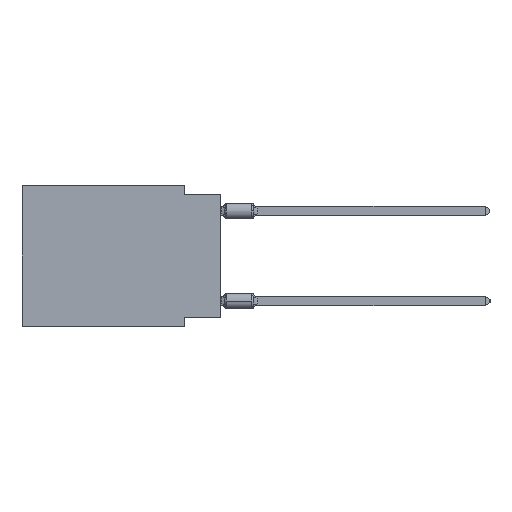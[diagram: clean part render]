
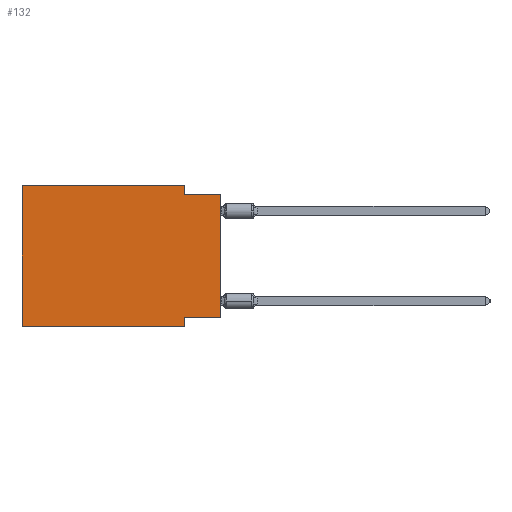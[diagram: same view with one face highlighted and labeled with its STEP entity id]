
A CAD part, left-side view. The second image highlights one B-rep face of the part: STEP entity #132.
In plain terms, the highlighted planar face has unit normal (-1, 0, 0).
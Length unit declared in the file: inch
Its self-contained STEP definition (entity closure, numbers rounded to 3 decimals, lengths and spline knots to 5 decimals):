
#132 = ADVANCED_FACE ( 'NONE', ( #26455 ), #16922, .F. ) ;
#209 = EDGE_CURVE ( 'NONE', #11832, #722, #6867, .T. ) ;
#321 = LINE ( 'NONE', #10527, #19018 ) ;
#358 = DIRECTION ( 'NONE',  ( 0., 0., -1. ) ) ;
#425 = CARTESIAN_POINT ( 'NONE',  ( 0., 0., -0.025 ) ) ;
#722 = VERTEX_POINT ( 'NONE', #29052 ) ;
#1105 = VECTOR ( 'NONE', #358, 39.37008 ) ;
#1753 = DIRECTION ( 'NONE',  ( 1., 0., 0. ) ) ;
#3013 = LINE ( 'NONE', #30524, #1105 ) ;
#3187 = CARTESIAN_POINT ( 'NONE',  ( 0., 0., -0.365 ) ) ;
#3414 = VERTEX_POINT ( 'NONE', #19768 ) ;
#3905 = CARTESIAN_POINT ( 'NONE',  ( 0., 0.55, 0. ) ) ;
#4203 = AXIS2_PLACEMENT_3D ( 'NONE', #3905, #1753, #29095 ) ;
#6547 = CARTESIAN_POINT ( 'NONE',  ( 0., 0.1, 0. ) ) ;
#6650 = ORIENTED_EDGE ( 'NONE', *, *, #29972, .F. ) ;
#6814 = ORIENTED_EDGE ( 'NONE', *, *, #30491, .F. ) ;
#6867 = LINE ( 'NONE', #6547, #7370 ) ;
#7124 = LINE ( 'NONE', #12048, #7965 ) ;
#7370 = VECTOR ( 'NONE', #11789, 39.37008 ) ;
#7598 = DIRECTION ( 'NONE',  ( 0., 0., 1. ) ) ;
#7965 = VECTOR ( 'NONE', #32156, 39.37008 ) ;
#8181 = ORIENTED_EDGE ( 'NONE', *, *, #19291, .F. ) ;
#8898 = VERTEX_POINT ( 'NONE', #12529 ) ;
#9011 = LINE ( 'NONE', #29116, #17925 ) ;
#10527 = CARTESIAN_POINT ( 'NONE',  ( 0., 0.55, 0. ) ) ;
#11071 = ORIENTED_EDGE ( 'NONE', *, *, #22305, .F. ) ;
#11384 = CARTESIAN_POINT ( 'NONE',  ( 0., 0., -0.025 ) ) ;
#11789 = DIRECTION ( 'NONE',  ( 0., 0., -1. ) ) ;
#11832 = VERTEX_POINT ( 'NONE', #28948 ) ;
#12048 = CARTESIAN_POINT ( 'NONE',  ( 0., 0.55, 0. ) ) ;
#12141 = CARTESIAN_POINT ( 'NONE',  ( 0., 0.55, 0. ) ) ;
#12402 = EDGE_LOOP ( 'NONE', ( #16361, #20812, #17800, #11071, #6814, #16056, #6650, #8181 ) ) ;
#12529 = CARTESIAN_POINT ( 'NONE',  ( 0., 0.1, -0.365 ) ) ;
#13703 = VERTEX_POINT ( 'NONE', #3187 ) ;
#15213 = VECTOR ( 'NONE', #16576, 39.37008 ) ;
#15964 = VERTEX_POINT ( 'NONE', #12141 ) ;
#16056 = ORIENTED_EDGE ( 'NONE', *, *, #26230, .T. ) ;
#16191 = DIRECTION ( 'NONE',  ( 0., -1., 0. ) ) ;
#16361 = ORIENTED_EDGE ( 'NONE', *, *, #21420, .T. ) ;
#16576 = DIRECTION ( 'NONE',  ( 0., 1., 0. ) ) ;
#16922 = PLANE ( 'NONE',  #4203 ) ;
#17800 = ORIENTED_EDGE ( 'NONE', *, *, #209, .F. ) ;
#17925 = VECTOR ( 'NONE', #30934, 39.37008 ) ;
#18170 = CARTESIAN_POINT ( 'NONE',  ( 0., 0.55, -0.39 ) ) ;
#19018 = VECTOR ( 'NONE', #7598, 39.37008 ) ;
#19291 = EDGE_CURVE ( 'NONE', #13703, #8898, #20976, .T. ) ;
#19711 = EDGE_CURVE ( 'NONE', #722, #26803, #27562, .T. ) ;
#19768 = CARTESIAN_POINT ( 'NONE',  ( 0., 0.1, -0.39 ) ) ;
#20812 = ORIENTED_EDGE ( 'NONE', *, *, #19711, .F. ) ;
#20976 = LINE ( 'NONE', #26251, #15213 ) ;
#21420 = EDGE_CURVE ( 'NONE', #13703, #26803, #9011, .T. ) ;
#21541 = VECTOR ( 'NONE', #16191, 39.37008 ) ;
#22305 = EDGE_CURVE ( 'NONE', #15964, #11832, #7124, .T. ) ;
#23339 = LINE ( 'NONE', #25177, #30691 ) ;
#25177 = CARTESIAN_POINT ( 'NONE',  ( 0., 0.55, -0.39 ) ) ;
#26230 = EDGE_CURVE ( 'NONE', #29979, #3414, #23339, .T. ) ;
#26251 = CARTESIAN_POINT ( 'NONE',  ( 0., 0., -0.365 ) ) ;
#26455 = FACE_OUTER_BOUND ( 'NONE', #12402, .T. ) ;
#26803 = VERTEX_POINT ( 'NONE', #425 ) ;
#27172 = DIRECTION ( 'NONE',  ( 0., -1., 0. ) ) ;
#27562 = LINE ( 'NONE', #11384, #21541 ) ;
#28948 = CARTESIAN_POINT ( 'NONE',  ( 0., 0.1, 0. ) ) ;
#29052 = CARTESIAN_POINT ( 'NONE',  ( 0., 0.1, -0.025 ) ) ;
#29095 = DIRECTION ( 'NONE',  ( 0., 0., -1. ) ) ;
#29116 = CARTESIAN_POINT ( 'NONE',  ( 0., 0., 0. ) ) ;
#29972 = EDGE_CURVE ( 'NONE', #8898, #3414, #3013, .T. ) ;
#29979 = VERTEX_POINT ( 'NONE', #18170 ) ;
#30491 = EDGE_CURVE ( 'NONE', #29979, #15964, #321, .T. ) ;
#30524 = CARTESIAN_POINT ( 'NONE',  ( 0., 0.1, -0.39 ) ) ;
#30691 = VECTOR ( 'NONE', #27172, 39.37008 ) ;
#30934 = DIRECTION ( 'NONE',  ( 0., 0., 1. ) ) ;
#32156 = DIRECTION ( 'NONE',  ( 0., -1., 0. ) ) ;
